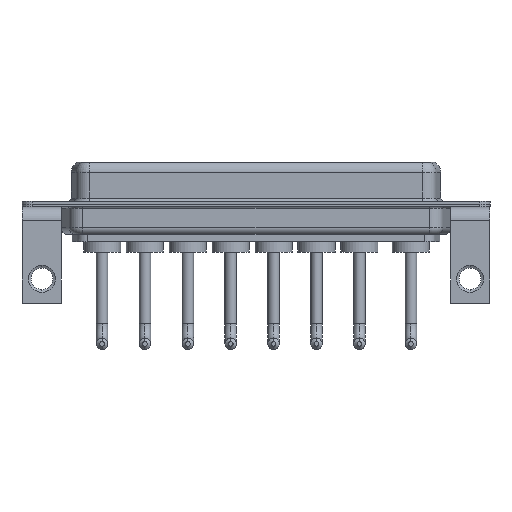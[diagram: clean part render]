
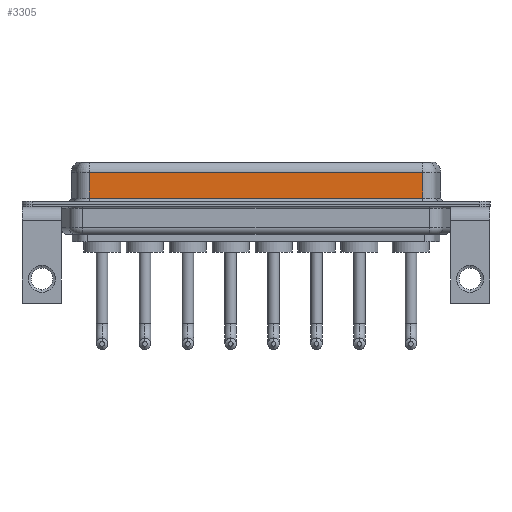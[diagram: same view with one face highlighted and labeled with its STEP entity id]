
A CAD part, front view. The second image highlights one B-rep face of the part: STEP entity #3305.
In plain terms, the highlighted planar face has unit normal (0, -1, 0).
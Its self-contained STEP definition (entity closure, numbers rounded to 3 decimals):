
#440 = DIRECTION ( 'NONE',  ( 0., 1., 0. ) ) ;
#1009 = DIRECTION ( 'NONE',  ( 0., 0., -1. ) ) ;
#1174 = VERTEX_POINT ( 'NONE', #8435 ) ;
#1313 = VERTEX_POINT ( 'NONE', #11763 ) ;
#1642 = VERTEX_POINT ( 'NONE', #2790 ) ;
#1960 = ORIENTED_EDGE ( 'NONE', *, *, #8847, .T. ) ;
#2007 = CARTESIAN_POINT ( 'NONE',  ( 56.462, -3.95, 6.4 ) ) ;
#2316 = VECTOR ( 'NONE', #3543, 1000. ) ;
#2790 = CARTESIAN_POINT ( 'NONE',  ( 7.038, -3.95, 0.9 ) ) ;
#3292 = CARTESIAN_POINT ( 'NONE',  ( 56.462, -3.95, 4.65 ) ) ;
#3305 = ADVANCED_FACE ( 'NONE', ( #8968 ), #10965, .F. ) ;
#3360 = DIRECTION ( 'NONE',  ( -1., 0., 0. ) ) ;
#3406 = CARTESIAN_POINT ( 'NONE',  ( 7.038, -3.95, 6.4 ) ) ;
#3543 = DIRECTION ( 'NONE',  ( 0., 0., -1. ) ) ;
#3705 = EDGE_CURVE ( 'NONE', #5441, #1642, #13139, .T. ) ;
#3710 = VECTOR ( 'NONE', #3360, 1000. ) ;
#3752 = LINE ( 'NONE', #10451, #6068 ) ;
#4386 = CARTESIAN_POINT ( 'NONE',  ( 7.038, -3.95, 4.65 ) ) ;
#4769 = DIRECTION ( 'NONE',  ( 0., 0., 1. ) ) ;
#5441 = VERTEX_POINT ( 'NONE', #4386 ) ;
#6068 = VECTOR ( 'NONE', #9375, 1000. ) ;
#6525 = EDGE_CURVE ( 'NONE', #1642, #1313, #3752, .T. ) ;
#7407 = ORIENTED_EDGE ( 'NONE', *, *, #6525, .T. ) ;
#8319 = ORIENTED_EDGE ( 'NONE', *, *, #3705, .T. ) ;
#8435 = CARTESIAN_POINT ( 'NONE',  ( 56.462, -3.95, 4.65 ) ) ;
#8847 = EDGE_CURVE ( 'NONE', #1174, #5441, #10968, .T. ) ;
#8968 = FACE_OUTER_BOUND ( 'NONE', #9496, .T. ) ;
#9099 = CARTESIAN_POINT ( 'NONE',  ( 56.462, -3.95, 6.4 ) ) ;
#9375 = DIRECTION ( 'NONE',  ( 1., 0., 0. ) ) ;
#9496 = EDGE_LOOP ( 'NONE', ( #11334, #1960, #8319, #7407 ) ) ;
#9803 = AXIS2_PLACEMENT_3D ( 'NONE', #9099, #440, #4769 ) ;
#10355 = VECTOR ( 'NONE', #1009, 1000. ) ;
#10451 = CARTESIAN_POINT ( 'NONE',  ( 56.462, -3.95, 0.9 ) ) ;
#10965 = PLANE ( 'NONE',  #9803 ) ;
#10968 = LINE ( 'NONE', #3292, #3710 ) ;
#11334 = ORIENTED_EDGE ( 'NONE', *, *, #12386, .F. ) ;
#11763 = CARTESIAN_POINT ( 'NONE',  ( 56.462, -3.95, 0.9 ) ) ;
#12386 = EDGE_CURVE ( 'NONE', #1174, #1313, #12998, .T. ) ;
#12998 = LINE ( 'NONE', #2007, #10355 ) ;
#13139 = LINE ( 'NONE', #3406, #2316 ) ;
